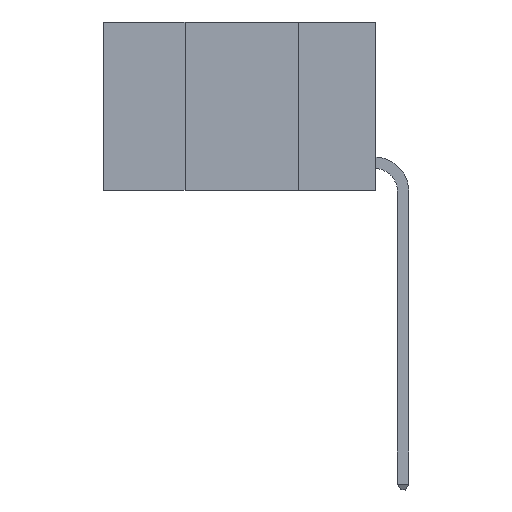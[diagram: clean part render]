
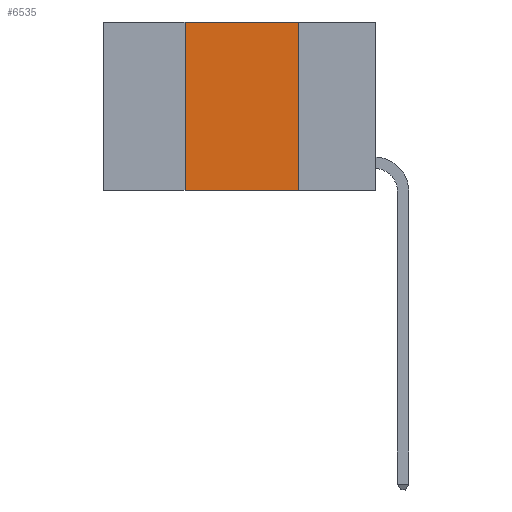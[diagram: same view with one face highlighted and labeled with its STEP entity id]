
A CAD part, left-side view. The second image highlights one B-rep face of the part: STEP entity #6535.
In plain terms, the highlighted planar face has unit normal (-1, 0, 0).
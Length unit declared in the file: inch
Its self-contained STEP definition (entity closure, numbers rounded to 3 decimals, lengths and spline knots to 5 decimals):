
#905 = VERTEX_POINT ( 'NONE', #984 ) ;
#984 = CARTESIAN_POINT ( 'NONE',  ( 0., 0.42, 0. ) ) ;
#1067 = PLANE ( 'NONE',  #6018 ) ;
#2409 = DIRECTION ( 'NONE',  ( 0., 0., 1. ) ) ;
#2500 = CARTESIAN_POINT ( 'NONE',  ( 0., 0.6, 0. ) ) ;
#2903 = VECTOR ( 'NONE', #15169, 39.37008 ) ;
#3689 = ORIENTED_EDGE ( 'NONE', *, *, #13100, .F. ) ;
#3933 = DIRECTION ( 'NONE',  ( 0., 0., -1. ) ) ;
#4647 = FACE_OUTER_BOUND ( 'NONE', #8888, .T. ) ;
#5964 = VERTEX_POINT ( 'NONE', #11558 ) ;
#6018 = AXIS2_PLACEMENT_3D ( 'NONE', #2500, #12626, #3933 ) ;
#6302 = EDGE_CURVE ( 'NONE', #7296, #13483, #15753, .T. ) ;
#6535 = ADVANCED_FACE ( 'NONE', ( #4647 ), #1067, .F. ) ;
#7296 = VERTEX_POINT ( 'NONE', #11462 ) ;
#8816 = VECTOR ( 'NONE', #10173, 39.37008 ) ;
#8888 = EDGE_LOOP ( 'NONE', ( #13679, #9365, #3689, #10956 ) ) ;
#9134 = DIRECTION ( 'NONE',  ( 0., -1., 0. ) ) ;
#9365 = ORIENTED_EDGE ( 'NONE', *, *, #12990, .F. ) ;
#10173 = DIRECTION ( 'NONE',  ( 0., 0., -1. ) ) ;
#10956 = ORIENTED_EDGE ( 'NONE', *, *, #6302, .T. ) ;
#11462 = CARTESIAN_POINT ( 'NONE',  ( 0., 0.42, -0.37 ) ) ;
#11558 = CARTESIAN_POINT ( 'NONE',  ( 0., 0.17, 0. ) ) ;
#11584 = CARTESIAN_POINT ( 'NONE',  ( 0., 0.17, 0. ) ) ;
#11729 = VECTOR ( 'NONE', #2409, 39.37008 ) ;
#11776 = EDGE_CURVE ( 'NONE', #5964, #13483, #12692, .T. ) ;
#12013 = CARTESIAN_POINT ( 'NONE',  ( 0., 0.17, -0.37 ) ) ;
#12626 = DIRECTION ( 'NONE',  ( 1., 0., 0. ) ) ;
#12692 = LINE ( 'NONE', #11584, #8816 ) ;
#12990 = EDGE_CURVE ( 'NONE', #905, #5964, #17831, .T. ) ;
#13100 = EDGE_CURVE ( 'NONE', #7296, #905, #16007, .T. ) ;
#13483 = VERTEX_POINT ( 'NONE', #12013 ) ;
#13679 = ORIENTED_EDGE ( 'NONE', *, *, #11776, .F. ) ;
#13728 = CARTESIAN_POINT ( 'NONE',  ( 0., 0.6, 0. ) ) ;
#14891 = CARTESIAN_POINT ( 'NONE',  ( 0., 0.6, -0.37 ) ) ;
#15169 = DIRECTION ( 'NONE',  ( 0., -1., 0. ) ) ;
#15753 = LINE ( 'NONE', #14891, #18711 ) ;
#16007 = LINE ( 'NONE', #16867, #11729 ) ;
#16867 = CARTESIAN_POINT ( 'NONE',  ( 0., 0.42, 0. ) ) ;
#17831 = LINE ( 'NONE', #13728, #2903 ) ;
#18711 = VECTOR ( 'NONE', #9134, 39.37008 ) ;
